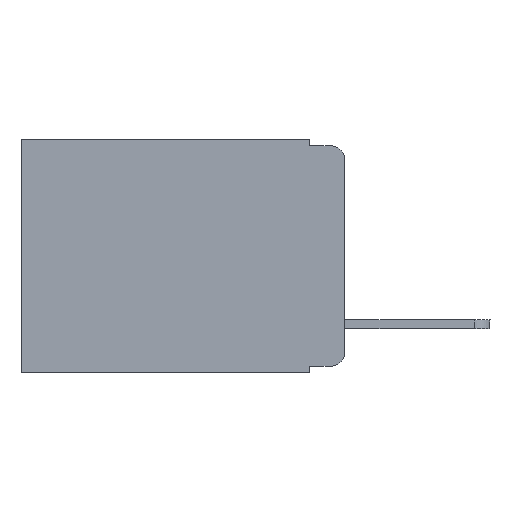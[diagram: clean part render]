
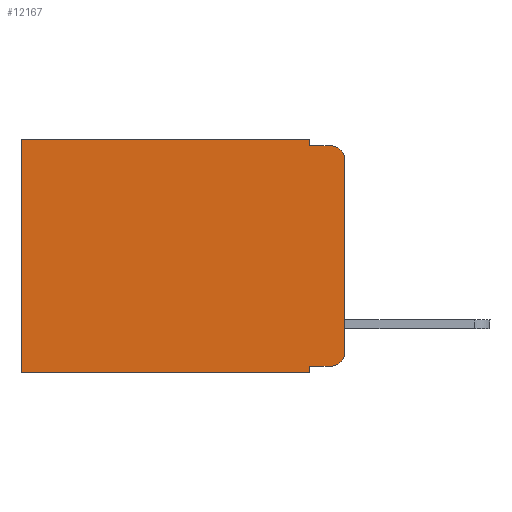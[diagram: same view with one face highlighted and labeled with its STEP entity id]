
A CAD part, left-side view. The second image highlights one B-rep face of the part: STEP entity #12167.
In plain terms, the highlighted planar face has unit normal (-1, 0, 0).
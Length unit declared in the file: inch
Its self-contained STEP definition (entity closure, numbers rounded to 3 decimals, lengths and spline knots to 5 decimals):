
#43 = LINE ( 'NONE', #6067, #3638 ) ;
#73 = VECTOR ( 'NONE', #7563, 39.37008 ) ;
#160 = AXIS2_PLACEMENT_3D ( 'NONE', #4070, #8058, #9230 ) ;
#416 = CARTESIAN_POINT ( 'NONE',  ( 0.298, 0.02, -0.01 ) ) ;
#488 = DIRECTION ( 'NONE',  ( -1., 0., 0. ) ) ;
#517 = VERTEX_POINT ( 'NONE', #1065 ) ;
#551 = VERTEX_POINT ( 'NONE', #8259 ) ;
#593 = LINE ( 'NONE', #4434, #2798 ) ;
#724 = DIRECTION ( 'NONE',  ( 0., 0., -1. ) ) ;
#742 = DIRECTION ( 'NONE',  ( 0., 0., -1. ) ) ;
#867 = VERTEX_POINT ( 'NONE', #5817 ) ;
#996 = CIRCLE ( 'NONE', #2258, 0.02 ) ;
#1065 = CARTESIAN_POINT ( 'NONE',  ( 0.298, 0.473, 0. ) ) ;
#1104 = DIRECTION ( 'NONE',  ( 0., 0., -1. ) ) ;
#1198 = VECTOR ( 'NONE', #742, 39.37008 ) ;
#1333 = CARTESIAN_POINT ( 'NONE',  ( 0.298, 0.051, 0. ) ) ;
#1530 = CARTESIAN_POINT ( 'NONE',  ( 0.298, 0.051, -0.333 ) ) ;
#1702 = EDGE_LOOP ( 'NONE', ( #7118, #4545, #10230, #12024, #10141, #10201, #4140, #6893, #11425, #11434 ) ) ;
#1957 = VERTEX_POINT ( 'NONE', #1530 ) ;
#2258 = AXIS2_PLACEMENT_3D ( 'NONE', #5440, #488, #12583 ) ;
#2367 = EDGE_CURVE ( 'NONE', #517, #10511, #593, .T. ) ;
#2798 = VECTOR ( 'NONE', #6404, 39.37008 ) ;
#2839 = AXIS2_PLACEMENT_3D ( 'NONE', #3728, #5811, #724 ) ;
#3433 = VECTOR ( 'NONE', #6554, 39.37008 ) ;
#3556 = CARTESIAN_POINT ( 'NONE',  ( 0.298, 0., 0. ) ) ;
#3638 = VECTOR ( 'NONE', #1104, 39.37008 ) ;
#3728 = CARTESIAN_POINT ( 'NONE',  ( 0.298, 0.02, -0.03 ) ) ;
#3943 = CARTESIAN_POINT ( 'NONE',  ( 0.298, 0., -0.313 ) ) ;
#3965 = DIRECTION ( 'NONE',  ( 0., -1., 0. ) ) ;
#4070 = CARTESIAN_POINT ( 'NONE',  ( 0.298, 0., 0. ) ) ;
#4124 = CARTESIAN_POINT ( 'NONE',  ( 0.298, 0.051, -0.01 ) ) ;
#4140 = ORIENTED_EDGE ( 'NONE', *, *, #8477, .F. ) ;
#4224 = CARTESIAN_POINT ( 'NONE',  ( 0.298, 0.02, -0.333 ) ) ;
#4248 = PLANE ( 'NONE',  #160 ) ;
#4434 = CARTESIAN_POINT ( 'NONE',  ( 0.298, 0.473, 0. ) ) ;
#4545 = ORIENTED_EDGE ( 'NONE', *, *, #10341, .T. ) ;
#4692 = VERTEX_POINT ( 'NONE', #4224 ) ;
#5112 = CARTESIAN_POINT ( 'NONE',  ( 0.298, 0.051, -0.333 ) ) ;
#5300 = CARTESIAN_POINT ( 'NONE',  ( 0.298, 0.051, 0. ) ) ;
#5305 = CARTESIAN_POINT ( 'NONE',  ( 0.298, 0., -0.343 ) ) ;
#5440 = CARTESIAN_POINT ( 'NONE',  ( 0.298, 0.02, -0.313 ) ) ;
#5552 = VERTEX_POINT ( 'NONE', #5300 ) ;
#5708 = LINE ( 'NONE', #12528, #73 ) ;
#5811 = DIRECTION ( 'NONE',  ( -1., 0., 0. ) ) ;
#5817 = CARTESIAN_POINT ( 'NONE',  ( 0.298, 0.051, -0.343 ) ) ;
#6023 = FACE_OUTER_BOUND ( 'NONE', #1702, .T. ) ;
#6067 = CARTESIAN_POINT ( 'NONE',  ( 0.298, 0.051, 0. ) ) ;
#6361 = LINE ( 'NONE', #5305, #3433 ) ;
#6404 = DIRECTION ( 'NONE',  ( 0., 0., -1. ) ) ;
#6478 = EDGE_CURVE ( 'NONE', #5552, #8692, #43, .T. ) ;
#6492 = EDGE_CURVE ( 'NONE', #5552, #517, #5708, .T. ) ;
#6554 = DIRECTION ( 'NONE',  ( 0., 1., 0. ) ) ;
#6718 = VERTEX_POINT ( 'NONE', #3943 ) ;
#6778 = EDGE_CURVE ( 'NONE', #1957, #867, #8326, .T. ) ;
#6893 = ORIENTED_EDGE ( 'NONE', *, *, #6778, .F. ) ;
#7118 = ORIENTED_EDGE ( 'NONE', *, *, #11549, .F. ) ;
#7232 = CIRCLE ( 'NONE', #2839, 0.02 ) ;
#7428 = EDGE_CURVE ( 'NONE', #8692, #8423, #12941, .T. ) ;
#7563 = DIRECTION ( 'NONE',  ( 0., 1., 0. ) ) ;
#7836 = CARTESIAN_POINT ( 'NONE',  ( 0.298, 0.051, -0.01 ) ) ;
#7879 = DIRECTION ( 'NONE',  ( 0., -1., 0. ) ) ;
#8058 = DIRECTION ( 'NONE',  ( 1., 0., 0. ) ) ;
#8259 = CARTESIAN_POINT ( 'NONE',  ( 0.298, 0., -0.03 ) ) ;
#8326 = LINE ( 'NONE', #1333, #9049 ) ;
#8423 = VERTEX_POINT ( 'NONE', #416 ) ;
#8477 = EDGE_CURVE ( 'NONE', #867, #10511, #6361, .T. ) ;
#8692 = VERTEX_POINT ( 'NONE', #4124 ) ;
#9049 = VECTOR ( 'NONE', #11213, 39.37008 ) ;
#9230 = DIRECTION ( 'NONE',  ( 0., 0., -1. ) ) ;
#10030 = LINE ( 'NONE', #5112, #12695 ) ;
#10097 = VECTOR ( 'NONE', #3965, 39.37008 ) ;
#10141 = ORIENTED_EDGE ( 'NONE', *, *, #6492, .T. ) ;
#10201 = ORIENTED_EDGE ( 'NONE', *, *, #2367, .T. ) ;
#10230 = ORIENTED_EDGE ( 'NONE', *, *, #7428, .F. ) ;
#10341 = EDGE_CURVE ( 'NONE', #551, #8423, #7232, .T. ) ;
#10511 = VERTEX_POINT ( 'NONE', #11190 ) ;
#11190 = CARTESIAN_POINT ( 'NONE',  ( 0.298, 0.473, -0.343 ) ) ;
#11213 = DIRECTION ( 'NONE',  ( 0., 0., -1. ) ) ;
#11323 = EDGE_CURVE ( 'NONE', #1957, #4692, #10030, .T. ) ;
#11425 = ORIENTED_EDGE ( 'NONE', *, *, #11323, .T. ) ;
#11434 = ORIENTED_EDGE ( 'NONE', *, *, #11901, .T. ) ;
#11549 = EDGE_CURVE ( 'NONE', #551, #6718, #11732, .T. ) ;
#11732 = LINE ( 'NONE', #3556, #1198 ) ;
#11901 = EDGE_CURVE ( 'NONE', #4692, #6718, #996, .T. ) ;
#12024 = ORIENTED_EDGE ( 'NONE', *, *, #6478, .F. ) ;
#12167 = ADVANCED_FACE ( 'NONE', ( #6023 ), #4248, .F. ) ;
#12528 = CARTESIAN_POINT ( 'NONE',  ( 0.298, 0., 0. ) ) ;
#12583 = DIRECTION ( 'NONE',  ( 0., 0., -1. ) ) ;
#12695 = VECTOR ( 'NONE', #7879, 39.37008 ) ;
#12941 = LINE ( 'NONE', #7836, #10097 ) ;
